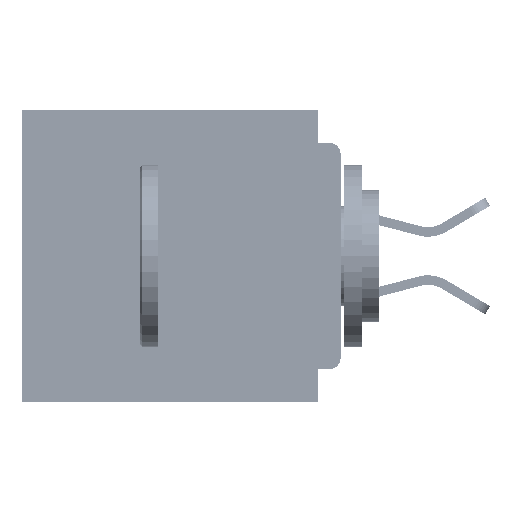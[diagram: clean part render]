
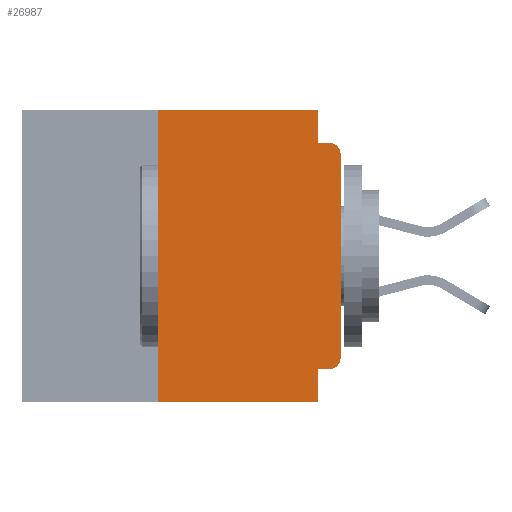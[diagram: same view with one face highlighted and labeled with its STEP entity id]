
A CAD part, left-side view. The second image highlights one B-rep face of the part: STEP entity #26987.
In plain terms, the highlighted planar face has unit normal (-1, 0, 0).
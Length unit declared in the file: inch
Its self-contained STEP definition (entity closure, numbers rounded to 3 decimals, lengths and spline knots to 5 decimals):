
#852 = EDGE_CURVE ( 'NONE', #40918, #51191, #10452, .T. ) ;
#1755 = EDGE_CURVE ( 'NONE', #51191, #13878, #10350, .T. ) ;
#2181 = VECTOR ( 'NONE', #8197, 39.37008 ) ;
#3213 = DIRECTION ( 'NONE',  ( 1., 0., 0. ) ) ;
#3666 = CARTESIAN_POINT ( 'NONE',  ( 0., 0.25, -0.4 ) ) ;
#5452 = CARTESIAN_POINT ( 'NONE',  ( 0., 0., 0. ) ) ;
#6022 = VERTEX_POINT ( 'NONE', #8183 ) ;
#6032 = VERTEX_POINT ( 'NONE', #12425 ) ;
#6597 = LINE ( 'NONE', #44357, #49919 ) ;
#8016 = LINE ( 'NONE', #52176, #27773 ) ;
#8183 = CARTESIAN_POINT ( 'NONE',  ( 0., 0.031, -0.045 ) ) ;
#8197 = DIRECTION ( 'NONE',  ( 0., 1., 0. ) ) ;
#8459 = ORIENTED_EDGE ( 'NONE', *, *, #50423, .F. ) ;
#9114 = VECTOR ( 'NONE', #51863, 39.37008 ) ;
#10350 = CIRCLE ( 'NONE', #34602, 0.015 ) ;
#10452 = LINE ( 'NONE', #5452, #9114 ) ;
#10878 = DIRECTION ( 'NONE',  ( 0., 0., -1. ) ) ;
#12425 = CARTESIAN_POINT ( 'NONE',  ( 0., 0.25, 0. ) ) ;
#12535 = ORIENTED_EDGE ( 'NONE', *, *, #24265, .F. ) ;
#12740 = CARTESIAN_POINT ( 'NONE',  ( 0., 0.015, -0.045 ) ) ;
#13198 = VERTEX_POINT ( 'NONE', #21115 ) ;
#13878 = VERTEX_POINT ( 'NONE', #12740 ) ;
#14753 = FACE_OUTER_BOUND ( 'NONE', #51481, .T. ) ;
#15830 = ORIENTED_EDGE ( 'NONE', *, *, #36008, .F. ) ;
#16247 = ORIENTED_EDGE ( 'NONE', *, *, #21220, .F. ) ;
#16846 = CIRCLE ( 'NONE', #19160, 0.015 ) ;
#17781 = CARTESIAN_POINT ( 'NONE',  ( 0., 0.25, -0.4 ) ) ;
#18094 = ORIENTED_EDGE ( 'NONE', *, *, #852, .T. ) ;
#18627 = LINE ( 'NONE', #47127, #50659 ) ;
#18969 = VERTEX_POINT ( 'NONE', #17781 ) ;
#19160 = AXIS2_PLACEMENT_3D ( 'NONE', #46141, #21136, #50352 ) ;
#19889 = ORIENTED_EDGE ( 'NONE', *, *, #41013, .F. ) ;
#20393 = CARTESIAN_POINT ( 'NONE',  ( 0., 0., -0.34 ) ) ;
#20942 = CARTESIAN_POINT ( 'NONE',  ( 0., 0., -0.355 ) ) ;
#21115 = CARTESIAN_POINT ( 'NONE',  ( 0., 0.031, 0. ) ) ;
#21136 = DIRECTION ( 'NONE',  ( -1., 0., 0. ) ) ;
#21220 = EDGE_CURVE ( 'NONE', #6032, #13198, #30000, .T. ) ;
#21891 = EDGE_CURVE ( 'NONE', #50188, #40918, #16846, .T. ) ;
#21974 = CARTESIAN_POINT ( 'NONE',  ( 0., 0.015, -0.355 ) ) ;
#22956 = DIRECTION ( 'NONE',  ( 0., -1., 0. ) ) ;
#23503 = CARTESIAN_POINT ( 'NONE',  ( 0., 0.031, -0.355 ) ) ;
#24265 = EDGE_CURVE ( 'NONE', #18969, #6032, #51053, .T. ) ;
#26987 = ADVANCED_FACE ( 'NONE', ( #14753 ), #37048, .F. ) ;
#27773 = VECTOR ( 'NONE', #22956, 39.37008 ) ;
#28534 = CARTESIAN_POINT ( 'NONE',  ( 0., 0.031, 0. ) ) ;
#28601 = EDGE_CURVE ( 'NONE', #18969, #46316, #18627, .T. ) ;
#28947 = DIRECTION ( 'NONE',  ( 0., 0., 1. ) ) ;
#30000 = LINE ( 'NONE', #45257, #39748 ) ;
#30241 = AXIS2_PLACEMENT_3D ( 'NONE', #32871, #3213, #41240 ) ;
#31031 = ORIENTED_EDGE ( 'NONE', *, *, #1755, .T. ) ;
#32871 = CARTESIAN_POINT ( 'NONE',  ( 0., 0.437, 0. ) ) ;
#34602 = AXIS2_PLACEMENT_3D ( 'NONE', #48992, #47291, #47223 ) ;
#36008 = EDGE_CURVE ( 'NONE', #6022, #13878, #8016, .T. ) ;
#37048 = PLANE ( 'NONE',  #30241 ) ;
#38891 = DIRECTION ( 'NONE',  ( 0., -1., 0. ) ) ;
#39748 = VECTOR ( 'NONE', #49313, 39.37008 ) ;
#40461 = VECTOR ( 'NONE', #28947, 39.37008 ) ;
#40756 = VERTEX_POINT ( 'NONE', #23503 ) ;
#40918 = VERTEX_POINT ( 'NONE', #20393 ) ;
#41013 = EDGE_CURVE ( 'NONE', #50188, #40756, #45593, .T. ) ;
#41240 = DIRECTION ( 'NONE',  ( 0., 0., -1. ) ) ;
#41421 = CARTESIAN_POINT ( 'NONE',  ( 0., 0.031, -0.4 ) ) ;
#43323 = LINE ( 'NONE', #28534, #54443 ) ;
#44357 = CARTESIAN_POINT ( 'NONE',  ( 0., 0.031, -0.4 ) ) ;
#45039 = ORIENTED_EDGE ( 'NONE', *, *, #21891, .T. ) ;
#45197 = CARTESIAN_POINT ( 'NONE',  ( 0., 0., -0.06 ) ) ;
#45257 = CARTESIAN_POINT ( 'NONE',  ( 0., 0.437, 0. ) ) ;
#45593 = LINE ( 'NONE', #20942, #2181 ) ;
#46141 = CARTESIAN_POINT ( 'NONE',  ( 0., 0.015, -0.34 ) ) ;
#46316 = VERTEX_POINT ( 'NONE', #41421 ) ;
#47127 = CARTESIAN_POINT ( 'NONE',  ( 0., 0.437, -0.4 ) ) ;
#47223 = DIRECTION ( 'NONE',  ( 0., 0., -1. ) ) ;
#47291 = DIRECTION ( 'NONE',  ( -1., 0., 0. ) ) ;
#48155 = ORIENTED_EDGE ( 'NONE', *, *, #28601, .T. ) ;
#48992 = CARTESIAN_POINT ( 'NONE',  ( 0., 0.015, -0.06 ) ) ;
#49313 = DIRECTION ( 'NONE',  ( 0., -1., 0. ) ) ;
#49919 = VECTOR ( 'NONE', #10878, 39.37008 ) ;
#50188 = VERTEX_POINT ( 'NONE', #21974 ) ;
#50352 = DIRECTION ( 'NONE',  ( 0., 0., -1. ) ) ;
#50423 = EDGE_CURVE ( 'NONE', #40756, #46316, #6597, .T. ) ;
#50523 = EDGE_CURVE ( 'NONE', #13198, #6022, #43323, .T. ) ;
#50659 = VECTOR ( 'NONE', #38891, 39.37008 ) ;
#50902 = ORIENTED_EDGE ( 'NONE', *, *, #50523, .F. ) ;
#51053 = LINE ( 'NONE', #3666, #40461 ) ;
#51191 = VERTEX_POINT ( 'NONE', #45197 ) ;
#51481 = EDGE_LOOP ( 'NONE', ( #18094, #31031, #15830, #50902, #16247, #12535, #48155, #8459, #19889, #45039 ) ) ;
#51863 = DIRECTION ( 'NONE',  ( 0., 0., 1. ) ) ;
#52176 = CARTESIAN_POINT ( 'NONE',  ( 0., 0., -0.045 ) ) ;
#53500 = DIRECTION ( 'NONE',  ( 0., 0., -1. ) ) ;
#54443 = VECTOR ( 'NONE', #53500, 39.37008 ) ;
